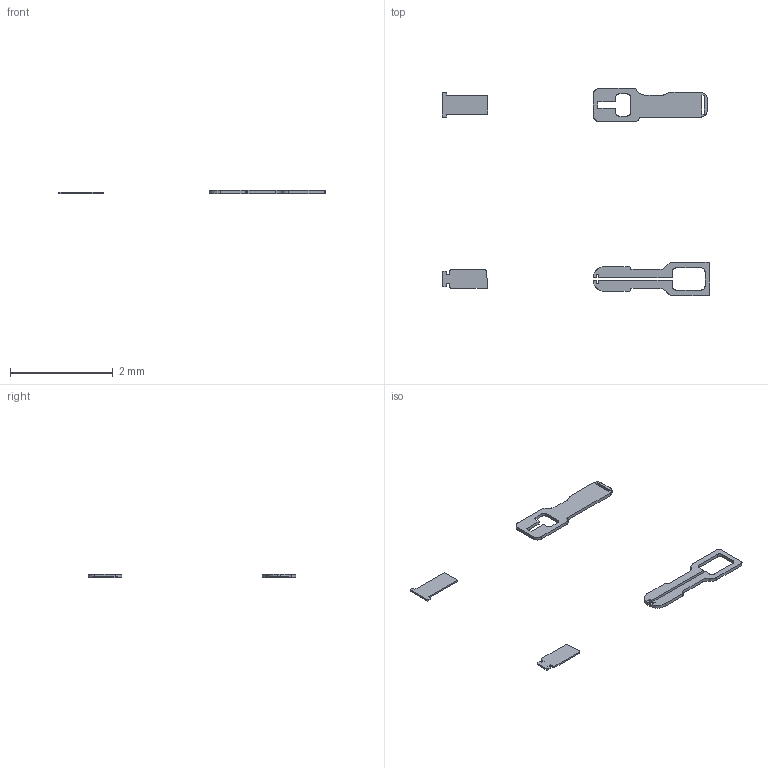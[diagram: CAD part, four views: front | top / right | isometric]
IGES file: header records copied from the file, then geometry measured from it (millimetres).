
Start section:  Autodesk DirectConnect version 5.0.70.0 ---- IGES version 5.3
Global section: file name: lightning link.iges; native system: Autodesk DirectConnect 5.0.70.0; preprocessor: 5.0.70.0; author: Deborah; organization: Unknown; date: 20130307.101842; units: millimetre
Bounding box: 5.21 x 4.04 x 0.06 mm (x, y, z)
Surface area: 6.2 mm2 (no closed solid volume)
Topology: 0 solids, 0 shells, 102 faces, 578 edges, 578 vertices
Faces by surface type: bspline 102
